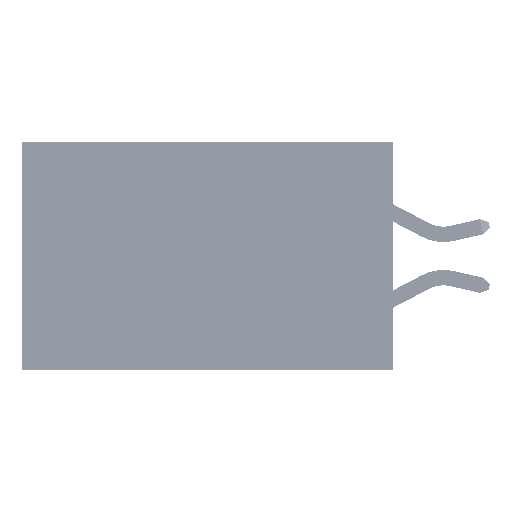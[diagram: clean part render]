
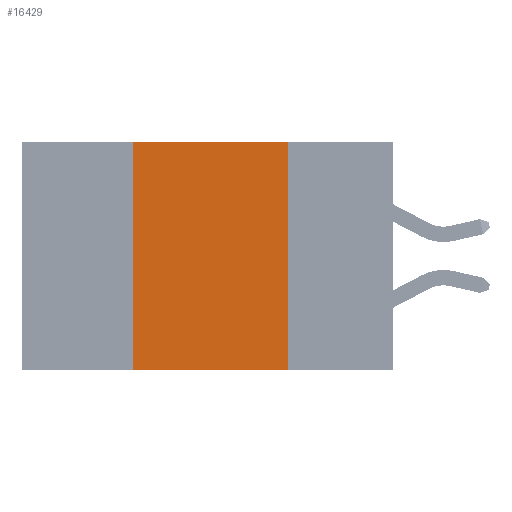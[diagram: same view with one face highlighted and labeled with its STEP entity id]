
A CAD part, left-side view. The second image highlights one B-rep face of the part: STEP entity #16429.
In plain terms, the highlighted planar face has unit normal (-1, 0, 0).
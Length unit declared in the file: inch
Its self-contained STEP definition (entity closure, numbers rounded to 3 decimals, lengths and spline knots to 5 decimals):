
#198 = DIRECTION ( 'NONE',  ( 0., 0., -1. ) ) ;
#627 = CARTESIAN_POINT ( 'NONE',  ( 0., 0.42, 0. ) ) ;
#2000 = CARTESIAN_POINT ( 'NONE',  ( 0., 0.42, -0.37 ) ) ;
#4386 = ORIENTED_EDGE ( 'NONE', *, *, #34318, .F. ) ;
#7580 = VECTOR ( 'NONE', #24452, 39.37008 ) ;
#9712 = VECTOR ( 'NONE', #27567, 39.37008 ) ;
#10549 = LINE ( 'NONE', #627, #23196 ) ;
#12269 = VERTEX_POINT ( 'NONE', #2000 ) ;
#12302 = DIRECTION ( 'NONE',  ( 1., 0., 0. ) ) ;
#13595 = LINE ( 'NONE', #13964, #30471 ) ;
#13964 = CARTESIAN_POINT ( 'NONE',  ( 0., 0.17, 0. ) ) ;
#16123 = ORIENTED_EDGE ( 'NONE', *, *, #38346, .T. ) ;
#16299 = CARTESIAN_POINT ( 'NONE',  ( 0., 0.17, -0.37 ) ) ;
#16429 = ADVANCED_FACE ( 'NONE', ( #37550 ), #32666, .F. ) ;
#16639 = VERTEX_POINT ( 'NONE', #16299 ) ;
#17445 = CARTESIAN_POINT ( 'NONE',  ( 0., 0.17, 0. ) ) ;
#19482 = EDGE_LOOP ( 'NONE', ( #38482, #43340, #4386, #16123 ) ) ;
#19744 = CARTESIAN_POINT ( 'NONE',  ( 0., 0.42, 0. ) ) ;
#19943 = VERTEX_POINT ( 'NONE', #19744 ) ;
#20653 = CARTESIAN_POINT ( 'NONE',  ( 0., 0.6, -0.37 ) ) ;
#23196 = VECTOR ( 'NONE', #37809, 39.37008 ) ;
#24452 = DIRECTION ( 'NONE',  ( 0., -1., 0. ) ) ;
#26594 = LINE ( 'NONE', #38002, #7580 ) ;
#27567 = DIRECTION ( 'NONE',  ( 0., -1., 0. ) ) ;
#28807 = DIRECTION ( 'NONE',  ( 0., 0., -1. ) ) ;
#28952 = AXIS2_PLACEMENT_3D ( 'NONE', #42840, #12302, #28807 ) ;
#30471 = VECTOR ( 'NONE', #198, 39.37008 ) ;
#32628 = EDGE_CURVE ( 'NONE', #19943, #33897, #26594, .T. ) ;
#32666 = PLANE ( 'NONE',  #28952 ) ;
#33897 = VERTEX_POINT ( 'NONE', #17445 ) ;
#34318 = EDGE_CURVE ( 'NONE', #12269, #19943, #10549, .T. ) ;
#36157 = EDGE_CURVE ( 'NONE', #33897, #16639, #13595, .T. ) ;
#37550 = FACE_OUTER_BOUND ( 'NONE', #19482, .T. ) ;
#37809 = DIRECTION ( 'NONE',  ( 0., 0., 1. ) ) ;
#38002 = CARTESIAN_POINT ( 'NONE',  ( 0., 0.6, 0. ) ) ;
#38346 = EDGE_CURVE ( 'NONE', #12269, #16639, #39218, .T. ) ;
#38482 = ORIENTED_EDGE ( 'NONE', *, *, #36157, .F. ) ;
#39218 = LINE ( 'NONE', #20653, #9712 ) ;
#42840 = CARTESIAN_POINT ( 'NONE',  ( 0., 0.6, 0. ) ) ;
#43340 = ORIENTED_EDGE ( 'NONE', *, *, #32628, .F. ) ;
